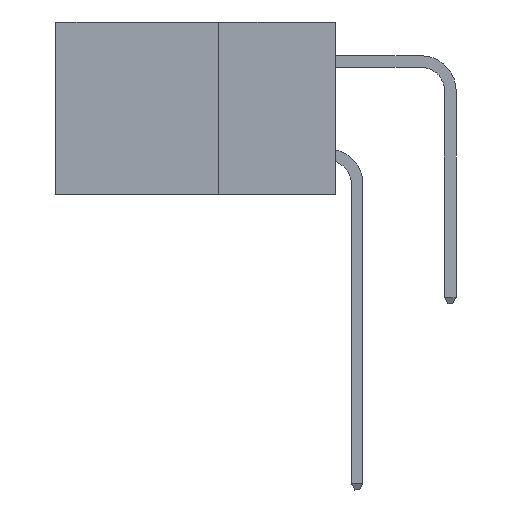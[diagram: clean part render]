
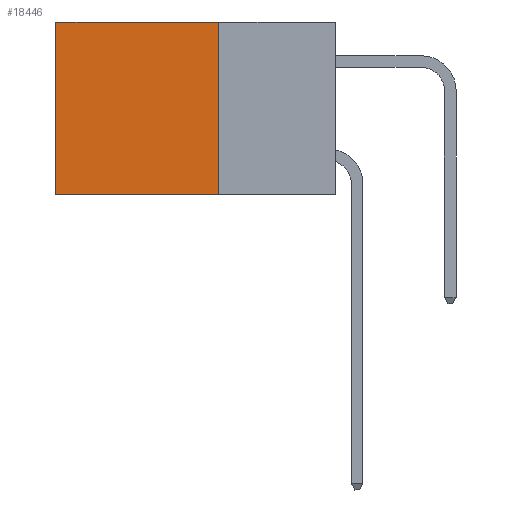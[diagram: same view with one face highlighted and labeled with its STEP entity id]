
A CAD part, left-side view. The second image highlights one B-rep face of the part: STEP entity #18446.
In plain terms, the highlighted planar face has unit normal (-1, 0, 0).
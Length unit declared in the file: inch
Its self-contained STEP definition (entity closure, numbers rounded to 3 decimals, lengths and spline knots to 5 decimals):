
#1063 = VECTOR ( 'NONE', #25375, 39.37008 ) ;
#1339 = VERTEX_POINT ( 'NONE', #31458 ) ;
#3222 = CARTESIAN_POINT ( 'NONE',  ( 0.2875, 0.25, 0. ) ) ;
#4590 = PLANE ( 'NONE',  #13563 ) ;
#4706 = DIRECTION ( 'NONE',  ( 1., 0., 0. ) ) ;
#5085 = EDGE_LOOP ( 'NONE', ( #20262, #20387, #16990, #23893 ) ) ;
#5925 = CARTESIAN_POINT ( 'NONE',  ( 0.2875, 0.25, 0. ) ) ;
#5932 = LINE ( 'NONE', #14859, #34902 ) ;
#10083 = DIRECTION ( 'NONE',  ( 0., 0., -1. ) ) ;
#11346 = LINE ( 'NONE', #24525, #28204 ) ;
#11810 = EDGE_CURVE ( 'NONE', #30927, #23565, #5932, .T. ) ;
#12333 = VECTOR ( 'NONE', #18268, 39.37008 ) ;
#13563 = AXIS2_PLACEMENT_3D ( 'NONE', #21170, #4706, #10083 ) ;
#14569 = EDGE_CURVE ( 'NONE', #33109, #1339, #11346, .T. ) ;
#14570 = FACE_OUTER_BOUND ( 'NONE', #5085, .T. ) ;
#14859 = CARTESIAN_POINT ( 'NONE',  ( 0.2875, 0.25, 0. ) ) ;
#16990 = ORIENTED_EDGE ( 'NONE', *, *, #24973, .F. ) ;
#18268 = DIRECTION ( 'NONE',  ( 0., 0., -1. ) ) ;
#18446 = ADVANCED_FACE ( 'NONE', ( #14570 ), #4590, .F. ) ;
#20262 = ORIENTED_EDGE ( 'NONE', *, *, #30048, .T. ) ;
#20387 = ORIENTED_EDGE ( 'NONE', *, *, #14569, .F. ) ;
#20424 = DIRECTION ( 'NONE',  ( 0., 1., 0. ) ) ;
#21170 = CARTESIAN_POINT ( 'NONE',  ( 0.2875, 0.25, 0. ) ) ;
#23565 = VERTEX_POINT ( 'NONE', #27043 ) ;
#23893 = ORIENTED_EDGE ( 'NONE', *, *, #11810, .T. ) ;
#24525 = CARTESIAN_POINT ( 'NONE',  ( 0.2875, 0.25, -0.37 ) ) ;
#24973 = EDGE_CURVE ( 'NONE', #30927, #33109, #35684, .T. ) ;
#25375 = DIRECTION ( 'NONE',  ( 0., 0., -1. ) ) ;
#27043 = CARTESIAN_POINT ( 'NONE',  ( 0.2875, 0.6, 0. ) ) ;
#28204 = VECTOR ( 'NONE', #30314, 39.37008 ) ;
#30048 = EDGE_CURVE ( 'NONE', #23565, #1339, #31349, .T. ) ;
#30314 = DIRECTION ( 'NONE',  ( 0., 1., 0. ) ) ;
#30927 = VERTEX_POINT ( 'NONE', #3222 ) ;
#31166 = CARTESIAN_POINT ( 'NONE',  ( 0.2875, 0.25, -0.37 ) ) ;
#31349 = LINE ( 'NONE', #35151, #12333 ) ;
#31458 = CARTESIAN_POINT ( 'NONE',  ( 0.2875, 0.6, -0.37 ) ) ;
#33109 = VERTEX_POINT ( 'NONE', #31166 ) ;
#34902 = VECTOR ( 'NONE', #20424, 39.37008 ) ;
#35151 = CARTESIAN_POINT ( 'NONE',  ( 0.2875, 0.6, 0. ) ) ;
#35684 = LINE ( 'NONE', #5925, #1063 ) ;
